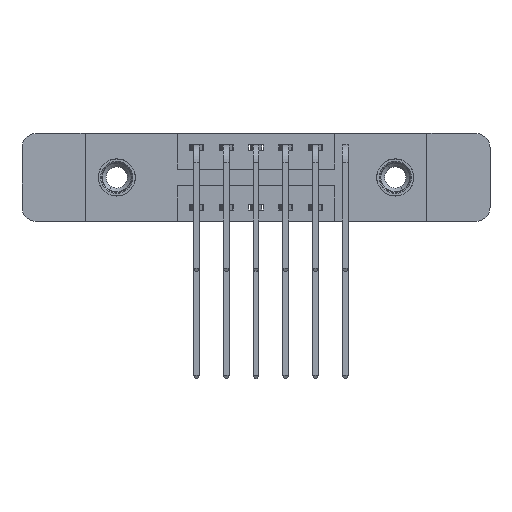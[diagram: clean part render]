
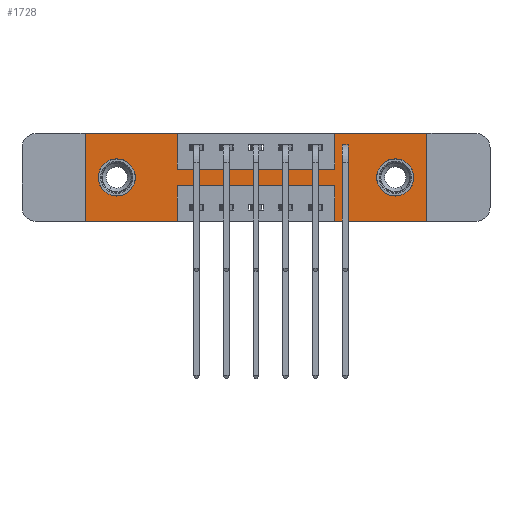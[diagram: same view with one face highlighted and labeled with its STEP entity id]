
A CAD part, front view. The second image highlights one B-rep face of the part: STEP entity #1728.
In plain terms, the highlighted planar face has unit normal (0, -1, 0).
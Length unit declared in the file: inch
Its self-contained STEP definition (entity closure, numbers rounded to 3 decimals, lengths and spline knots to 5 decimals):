
#95 = CARTESIAN_POINT ( 'NONE',  ( 0.3875, 0., -0.22 ) ) ;
#177 = ORIENTED_EDGE ( 'NONE', *, *, #13318, .F. ) ;
#279 = EDGE_LOOP ( 'NONE', ( #2688, #7151, #7759, #844, #4846, #8569, #5341, #11452, #177, #4757, #1811, #12397 ) ) ;
#362 = CARTESIAN_POINT ( 'NONE',  ( 0.3875, 0., -0.37 ) ) ;
#446 = VECTOR ( 'NONE', #3019, 39.37008 ) ;
#522 = EDGE_CURVE ( 'NONE', #12706, #8235, #10585, .T. ) ;
#541 = VECTOR ( 'NONE', #5194, 39.37008 ) ;
#618 = VECTOR ( 'NONE', #9157, 39.37008 ) ;
#718 = VECTOR ( 'NONE', #4061, 39.37008 ) ;
#785 = CARTESIAN_POINT ( 'NONE',  ( 0.1325, 0., -0.185 ) ) ;
#826 = DIRECTION ( 'NONE',  ( 0., 0., -1. ) ) ;
#840 = VECTOR ( 'NONE', #3906, 39.37008 ) ;
#844 = ORIENTED_EDGE ( 'NONE', *, *, #6543, .F. ) ;
#1095 = CARTESIAN_POINT ( 'NONE',  ( 0.3875, 0., 0. ) ) ;
#1151 = EDGE_CURVE ( 'NONE', #8600, #14738, #10422, .T. ) ;
#1259 = CARTESIAN_POINT ( 'NONE',  ( 1.0475, 0., 0. ) ) ;
#1290 = CARTESIAN_POINT ( 'NONE',  ( 1.3025, 0., -0.107 ) ) ;
#1422 = EDGE_CURVE ( 'NONE', #10020, #4112, #11257, .T. ) ;
#1432 = ORIENTED_EDGE ( 'NONE', *, *, #1151, .T. ) ;
#1518 = DIRECTION ( 'NONE',  ( -1., 0., 0. ) ) ;
#1644 = CARTESIAN_POINT ( 'NONE',  ( 0., 0., 0. ) ) ;
#1728 = ADVANCED_FACE ( 'NONE', ( #10108, #13666, #3094 ), #8975, .T. ) ;
#1811 = ORIENTED_EDGE ( 'NONE', *, *, #2555, .F. ) ;
#2040 = CARTESIAN_POINT ( 'NONE',  ( 0., 0., -0.37 ) ) ;
#2151 = DIRECTION ( 'NONE',  ( 0., 0., -1. ) ) ;
#2555 = EDGE_CURVE ( 'NONE', #3001, #12706, #12453, .T. ) ;
#2598 = LINE ( 'NONE', #12322, #11301 ) ;
#2688 = ORIENTED_EDGE ( 'NONE', *, *, #1422, .F. ) ;
#2717 = CARTESIAN_POINT ( 'NONE',  ( 1.0475, 0., -0.37 ) ) ;
#2775 = CARTESIAN_POINT ( 'NONE',  ( 0., 0., -0.37 ) ) ;
#2904 = CIRCLE ( 'NONE', #9502, 0.078 ) ;
#2961 = CIRCLE ( 'NONE', #3543, 0.078 ) ;
#3001 = VERTEX_POINT ( 'NONE', #2040 ) ;
#3019 = DIRECTION ( 'NONE',  ( 1., 0., 0. ) ) ;
#3094 = FACE_OUTER_BOUND ( 'NONE', #279, .T. ) ;
#3543 = AXIS2_PLACEMENT_3D ( 'NONE', #14159, #15435, #2151 ) ;
#3570 = AXIS2_PLACEMENT_3D ( 'NONE', #11835, #6735, #9108 ) ;
#3906 = DIRECTION ( 'NONE',  ( 0., 0., 1. ) ) ;
#3942 = CARTESIAN_POINT ( 'NONE',  ( 1.0475, 0., -0.22 ) ) ;
#3946 = CIRCLE ( 'NONE', #14357, 0.078 ) ;
#4061 = DIRECTION ( 'NONE',  ( -1., 0., 0. ) ) ;
#4112 = VERTEX_POINT ( 'NONE', #14361 ) ;
#4225 = CARTESIAN_POINT ( 'NONE',  ( 1.0475, 0., 0. ) ) ;
#4757 = ORIENTED_EDGE ( 'NONE', *, *, #522, .F. ) ;
#4836 = EDGE_CURVE ( 'NONE', #13360, #7033, #6532, .T. ) ;
#4846 = ORIENTED_EDGE ( 'NONE', *, *, #9984, .F. ) ;
#5016 = LINE ( 'NONE', #95, #718 ) ;
#5080 = EDGE_LOOP ( 'NONE', ( #10028, #13956 ) ) ;
#5194 = DIRECTION ( 'NONE',  ( 0., 0., -1. ) ) ;
#5240 = VECTOR ( 'NONE', #9078, 39.37008 ) ;
#5288 = CARTESIAN_POINT ( 'NONE',  ( 1.435, 0., -0.37 ) ) ;
#5341 = ORIENTED_EDGE ( 'NONE', *, *, #7659, .F. ) ;
#5503 = CARTESIAN_POINT ( 'NONE',  ( 0.3875, 0., -0.22 ) ) ;
#5556 = LINE ( 'NONE', #7721, #446 ) ;
#5574 = CARTESIAN_POINT ( 'NONE',  ( 0.3875, 0., 0. ) ) ;
#5849 = VECTOR ( 'NONE', #8750, 39.37008 ) ;
#6214 = CARTESIAN_POINT ( 'NONE',  ( 0., 0., 0. ) ) ;
#6279 = DIRECTION ( 'NONE',  ( -1., 0., 0. ) ) ;
#6394 = DIRECTION ( 'NONE',  ( 0., 0., 1. ) ) ;
#6435 = DIRECTION ( 'NONE',  ( 0., -1., 0. ) ) ;
#6532 = LINE ( 'NONE', #2717, #840 ) ;
#6543 = EDGE_CURVE ( 'NONE', #12448, #13360, #11380, .T. ) ;
#6735 = DIRECTION ( 'NONE',  ( 0., 1., 0. ) ) ;
#6862 = VECTOR ( 'NONE', #6394, 39.37008 ) ;
#7033 = VERTEX_POINT ( 'NONE', #3942 ) ;
#7151 = ORIENTED_EDGE ( 'NONE', *, *, #10330, .F. ) ;
#7659 = EDGE_CURVE ( 'NONE', #7811, #13850, #12516, .T. ) ;
#7721 = CARTESIAN_POINT ( 'NONE',  ( 0.3875, 0., -0.15 ) ) ;
#7759 = ORIENTED_EDGE ( 'NONE', *, *, #4836, .F. ) ;
#7811 = VERTEX_POINT ( 'NONE', #8360 ) ;
#7947 = DIRECTION ( 'NONE',  ( 0., 0., -1. ) ) ;
#8047 = VERTEX_POINT ( 'NONE', #12476 ) ;
#8054 = VERTEX_POINT ( 'NONE', #1290 ) ;
#8122 = CARTESIAN_POINT ( 'NONE',  ( 0., 0., 0. ) ) ;
#8235 = VERTEX_POINT ( 'NONE', #1095 ) ;
#8360 = CARTESIAN_POINT ( 'NONE',  ( 1.0475, 0., -0.15 ) ) ;
#8519 = LINE ( 'NONE', #6214, #5849 ) ;
#8569 = ORIENTED_EDGE ( 'NONE', *, *, #10871, .F. ) ;
#8600 = VERTEX_POINT ( 'NONE', #12125 ) ;
#8713 = CARTESIAN_POINT ( 'NONE',  ( 0., 0., 0. ) ) ;
#8750 = DIRECTION ( 'NONE',  ( 1., 0., 0. ) ) ;
#8892 = VERTEX_POINT ( 'NONE', #10429 ) ;
#8975 = PLANE ( 'NONE',  #13988 ) ;
#9078 = DIRECTION ( 'NONE',  ( 0., 0., 1. ) ) ;
#9108 = DIRECTION ( 'NONE',  ( 0., 0., 1. ) ) ;
#9157 = DIRECTION ( 'NONE',  ( 0., 0., -1. ) ) ;
#9278 = DIRECTION ( 'NONE',  ( 0., 0., 1. ) ) ;
#9313 = DIRECTION ( 'NONE',  ( 0., 0., -1. ) ) ;
#9502 = AXIS2_PLACEMENT_3D ( 'NONE', #13710, #12905, #9313 ) ;
#9984 = EDGE_CURVE ( 'NONE', #8892, #12448, #15050, .T. ) ;
#10020 = VERTEX_POINT ( 'NONE', #5503 ) ;
#10028 = ORIENTED_EDGE ( 'NONE', *, *, #10584, .T. ) ;
#10108 = FACE_BOUND ( 'NONE', #5080, .T. ) ;
#10330 = EDGE_CURVE ( 'NONE', #7033, #10020, #5016, .T. ) ;
#10422 = CIRCLE ( 'NONE', #3570, 0.078 ) ;
#10429 = CARTESIAN_POINT ( 'NONE',  ( 1.435, 0., 0. ) ) ;
#10431 = LINE ( 'NONE', #5574, #618 ) ;
#10584 = EDGE_CURVE ( 'NONE', #8054, #8047, #2961, .T. ) ;
#10585 = LINE ( 'NONE', #8122, #11435 ) ;
#10871 = EDGE_CURVE ( 'NONE', #13850, #8892, #8519, .T. ) ;
#11039 = VECTOR ( 'NONE', #826, 39.37008 ) ;
#11063 = ORIENTED_EDGE ( 'NONE', *, *, #14791, .T. ) ;
#11257 = LINE ( 'NONE', #362, #541 ) ;
#11301 = VECTOR ( 'NONE', #6279, 39.37008 ) ;
#11380 = LINE ( 'NONE', #13663, #12815 ) ;
#11435 = VECTOR ( 'NONE', #11635, 39.37008 ) ;
#11452 = ORIENTED_EDGE ( 'NONE', *, *, #11988, .F. ) ;
#11578 = EDGE_CURVE ( 'NONE', #8047, #8054, #2904, .T. ) ;
#11635 = DIRECTION ( 'NONE',  ( 1., 0., 0. ) ) ;
#11835 = CARTESIAN_POINT ( 'NONE',  ( 0.1325, 0., -0.185 ) ) ;
#11975 = DIRECTION ( 'NONE',  ( 0., 1., 0. ) ) ;
#11988 = EDGE_CURVE ( 'NONE', #12217, #7811, #5556, .T. ) ;
#12125 = CARTESIAN_POINT ( 'NONE',  ( 0.1325, 0., -0.263 ) ) ;
#12130 = CARTESIAN_POINT ( 'NONE',  ( 0.1325, 0., -0.107 ) ) ;
#12217 = VERTEX_POINT ( 'NONE', #15430 ) ;
#12322 = CARTESIAN_POINT ( 'NONE',  ( 0., 0., -0.37 ) ) ;
#12397 = ORIENTED_EDGE ( 'NONE', *, *, #13479, .F. ) ;
#12448 = VERTEX_POINT ( 'NONE', #5288 ) ;
#12453 = LINE ( 'NONE', #1644, #6862 ) ;
#12476 = CARTESIAN_POINT ( 'NONE',  ( 1.3025, 0., -0.263 ) ) ;
#12516 = LINE ( 'NONE', #4225, #5240 ) ;
#12706 = VERTEX_POINT ( 'NONE', #8713 ) ;
#12815 = VECTOR ( 'NONE', #1518, 39.37008 ) ;
#12827 = EDGE_LOOP ( 'NONE', ( #11063, #1432 ) ) ;
#12905 = DIRECTION ( 'NONE',  ( 0., 1., 0. ) ) ;
#12981 = CARTESIAN_POINT ( 'NONE',  ( 1.435, 0., 0. ) ) ;
#13318 = EDGE_CURVE ( 'NONE', #8235, #12217, #10431, .T. ) ;
#13360 = VERTEX_POINT ( 'NONE', #15532 ) ;
#13479 = EDGE_CURVE ( 'NONE', #4112, #3001, #2598, .T. ) ;
#13663 = CARTESIAN_POINT ( 'NONE',  ( 0., 0., -0.37 ) ) ;
#13666 = FACE_BOUND ( 'NONE', #12827, .T. ) ;
#13710 = CARTESIAN_POINT ( 'NONE',  ( 1.3025, 0., -0.185 ) ) ;
#13850 = VERTEX_POINT ( 'NONE', #1259 ) ;
#13956 = ORIENTED_EDGE ( 'NONE', *, *, #11578, .T. ) ;
#13988 = AXIS2_PLACEMENT_3D ( 'NONE', #2775, #6435, #7947 ) ;
#14159 = CARTESIAN_POINT ( 'NONE',  ( 1.3025, 0., -0.185 ) ) ;
#14357 = AXIS2_PLACEMENT_3D ( 'NONE', #785, #11975, #9278 ) ;
#14361 = CARTESIAN_POINT ( 'NONE',  ( 0.3875, 0., -0.37 ) ) ;
#14738 = VERTEX_POINT ( 'NONE', #12130 ) ;
#14791 = EDGE_CURVE ( 'NONE', #14738, #8600, #3946, .T. ) ;
#15050 = LINE ( 'NONE', #12981, #11039 ) ;
#15430 = CARTESIAN_POINT ( 'NONE',  ( 0.3875, 0., -0.15 ) ) ;
#15435 = DIRECTION ( 'NONE',  ( 0., 1., 0. ) ) ;
#15532 = CARTESIAN_POINT ( 'NONE',  ( 1.0475, 0., -0.37 ) ) ;
